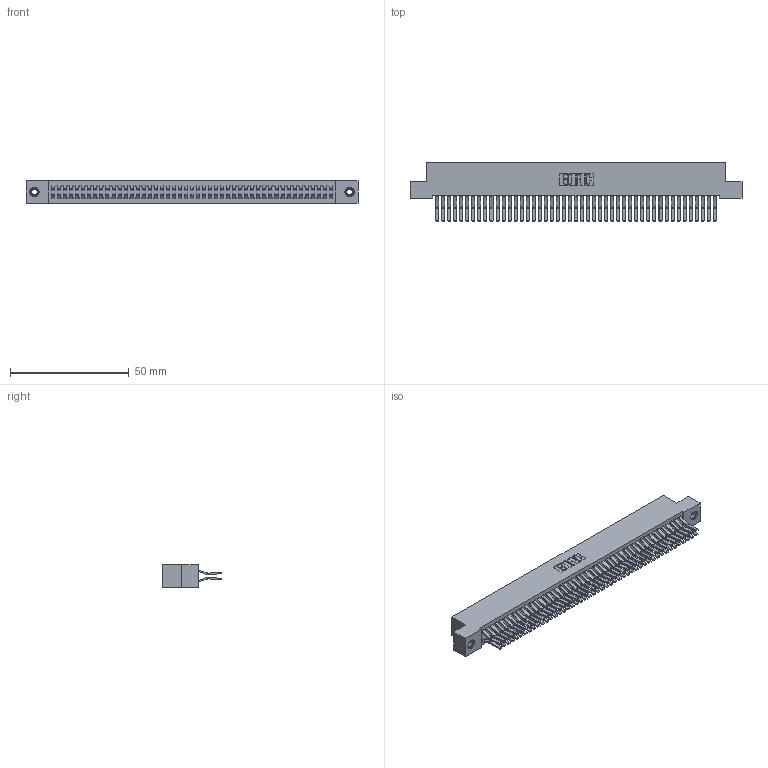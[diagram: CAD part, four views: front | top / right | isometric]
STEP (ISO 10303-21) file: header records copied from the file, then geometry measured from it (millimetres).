
FILE_DESCRIPTION (( 'STEP AP203' ), '1' );
FILE_NAME ('342-094-560-207.STEP', '2018-08-14T02:51:28', ( '' ), ( '' ), 'SwSTEP 2.0', 'SolidWorks 2016', '' );
FILE_SCHEMA (( 'CONFIG_CONTROL_DESIGN' ));
Length unit declared in the file: inch
Products named in the file (4): 342 Part_TI; 345-292-001_560 Tail; 345-250-001_345-250-005-103; 342-094-560-207
Assembly tree (97 placements, depth 2):
  342-094-560-207
    342 Part_TI
    345-292-001_560 Tail  x94
    345-250-001_345-250-005-103  x2
Bounding box: 139.7 x 24.78 x 9.4 mm (x, y, z)
Volume: 13180.1 mm3; surface area: 23082.8 mm2
Topology: 97 solids, 97 shells, 5246 faces, 15569 edges, 10246 vertices
Faces by surface type: plane 3482, cylinder 1748, cone 12, torus 4
Entity records: 30732 total; most frequent: CARTESIAN_POINT 5069, ORIENTED_EDGE 4998, DIRECTION 4357, EDGE_CURVE 2499, LINE 2347, VECTOR 2347, VERTEX_POINT 1660, AXIS2_PLACEMENT_3D 1005
